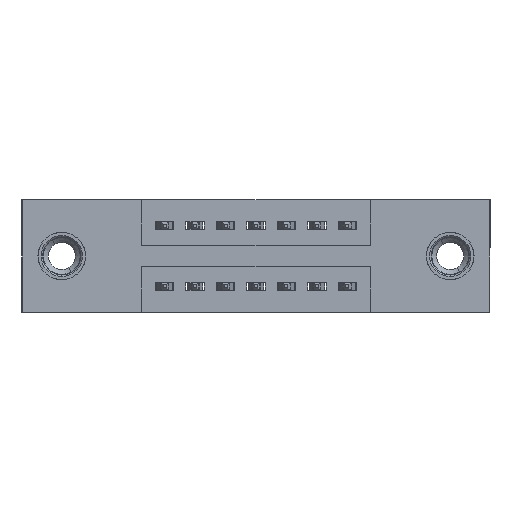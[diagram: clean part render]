
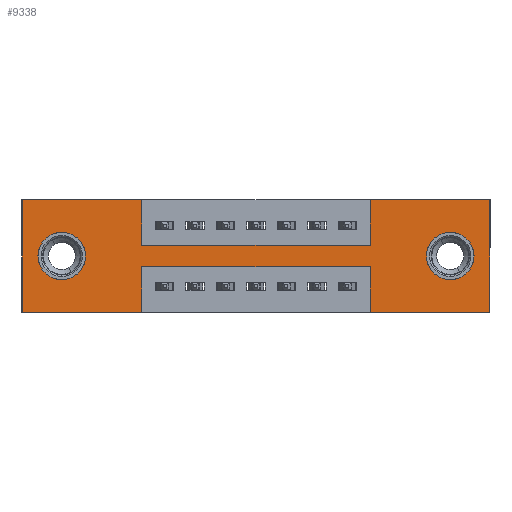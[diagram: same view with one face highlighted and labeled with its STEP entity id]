
A CAD part, front view. The second image highlights one B-rep face of the part: STEP entity #9338.
In plain terms, the highlighted planar face has unit normal (0, -1, 0).
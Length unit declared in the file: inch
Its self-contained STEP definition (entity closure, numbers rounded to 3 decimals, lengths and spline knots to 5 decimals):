
#310 = DIRECTION ( 'NONE',  ( 0., 1., 0. ) ) ;
#354 = LINE ( 'NONE', #8380, #3101 ) ;
#454 = CARTESIAN_POINT ( 'NONE',  ( 0.3925, 0., 0. ) ) ;
#519 = FACE_BOUND ( 'NONE', #1555, .T. ) ;
#572 = ORIENTED_EDGE ( 'NONE', *, *, #2110, .T. ) ;
#616 = CARTESIAN_POINT ( 'NONE',  ( 1.535, 0., -0.37 ) ) ;
#624 = LINE ( 'NONE', #11600, #9513 ) ;
#793 = VERTEX_POINT ( 'NONE', #9125 ) ;
#944 = ORIENTED_EDGE ( 'NONE', *, *, #11783, .F. ) ;
#978 = DIRECTION ( 'NONE',  ( 0., 1., 0. ) ) ;
#1040 = VERTEX_POINT ( 'NONE', #5684 ) ;
#1214 = DIRECTION ( 'NONE',  ( 0., 0., -1. ) ) ;
#1364 = AXIS2_PLACEMENT_3D ( 'NONE', #6795, #3445, #2253 ) ;
#1555 = EDGE_LOOP ( 'NONE', ( #9147, #572 ) ) ;
#1647 = VECTOR ( 'NONE', #11703, 39.37008 ) ;
#1664 = VECTOR ( 'NONE', #3648, 39.37008 ) ;
#1700 = CIRCLE ( 'NONE', #11660, 0.078 ) ;
#1796 = VERTEX_POINT ( 'NONE', #5261 ) ;
#1831 = CIRCLE ( 'NONE', #1364, 0.078 ) ;
#1840 = EDGE_CURVE ( 'NONE', #13525, #9590, #12715, .T. ) ;
#2037 = EDGE_CURVE ( 'NONE', #6480, #1040, #12182, .T. ) ;
#2058 = CARTESIAN_POINT ( 'NONE',  ( 0.13, 0., -0.185 ) ) ;
#2110 = EDGE_CURVE ( 'NONE', #3504, #793, #1831, .T. ) ;
#2253 = DIRECTION ( 'NONE',  ( 0., 0., -1. ) ) ;
#2272 = ORIENTED_EDGE ( 'NONE', *, *, #5285, .F. ) ;
#2352 = VECTOR ( 'NONE', #1214, 39.37008 ) ;
#2483 = ORIENTED_EDGE ( 'NONE', *, *, #1840, .F. ) ;
#2547 = ORIENTED_EDGE ( 'NONE', *, *, #14667, .F. ) ;
#2696 = VERTEX_POINT ( 'NONE', #13065 ) ;
#2777 = CARTESIAN_POINT ( 'NONE',  ( 0., 0., -0.37 ) ) ;
#3079 = DIRECTION ( 'NONE',  ( 0., 1., 0. ) ) ;
#3101 = VECTOR ( 'NONE', #11606, 39.37008 ) ;
#3163 = CARTESIAN_POINT ( 'NONE',  ( 0.3925, 0., -0.22 ) ) ;
#3194 = DIRECTION ( 'NONE',  ( 0., 0., -1. ) ) ;
#3234 = DIRECTION ( 'NONE',  ( 0., 0., 1. ) ) ;
#3445 = DIRECTION ( 'NONE',  ( 0., 1., 0. ) ) ;
#3475 = VECTOR ( 'NONE', #5201, 39.37008 ) ;
#3504 = VERTEX_POINT ( 'NONE', #3774 ) ;
#3574 = CARTESIAN_POINT ( 'NONE',  ( 1.1425, 0., 0. ) ) ;
#3644 = DIRECTION ( 'NONE',  ( -1., 0., 0. ) ) ;
#3648 = DIRECTION ( 'NONE',  ( 1., 0., 0. ) ) ;
#3651 = CARTESIAN_POINT ( 'NONE',  ( 1.535, 0., 0. ) ) ;
#3675 = VECTOR ( 'NONE', #5371, 39.37008 ) ;
#3748 = VERTEX_POINT ( 'NONE', #454 ) ;
#3774 = CARTESIAN_POINT ( 'NONE',  ( 1.405, 0., -0.263 ) ) ;
#3895 = CARTESIAN_POINT ( 'NONE',  ( 0.13, 0., -0.185 ) ) ;
#4017 = VECTOR ( 'NONE', #12720, 39.37008 ) ;
#4092 = VECTOR ( 'NONE', #9627, 39.37008 ) ;
#4129 = ORIENTED_EDGE ( 'NONE', *, *, #4266, .F. ) ;
#4266 = EDGE_CURVE ( 'NONE', #1796, #6480, #4285, .T. ) ;
#4283 = VECTOR ( 'NONE', #3194, 39.37008 ) ;
#4285 = LINE ( 'NONE', #3574, #9907 ) ;
#4526 = ORIENTED_EDGE ( 'NONE', *, *, #2037, .F. ) ;
#4536 = ORIENTED_EDGE ( 'NONE', *, *, #6891, .F. ) ;
#4721 = LINE ( 'NONE', #9426, #1647 ) ;
#4742 = DIRECTION ( 'NONE',  ( 0., 0., 1. ) ) ;
#4751 = CARTESIAN_POINT ( 'NONE',  ( 0.3925, 0., -0.15 ) ) ;
#4876 = ORIENTED_EDGE ( 'NONE', *, *, #11147, .F. ) ;
#4954 = CARTESIAN_POINT ( 'NONE',  ( 0.3925, 0., 0. ) ) ;
#5201 = DIRECTION ( 'NONE',  ( -1., 0., 0. ) ) ;
#5261 = CARTESIAN_POINT ( 'NONE',  ( 1.1425, 0., -0.15 ) ) ;
#5285 = EDGE_CURVE ( 'NONE', #11711, #9975, #624, .T. ) ;
#5316 = CARTESIAN_POINT ( 'NONE',  ( 0., 0., -0.37 ) ) ;
#5371 = DIRECTION ( 'NONE',  ( -1., 0., 0. ) ) ;
#5490 = LINE ( 'NONE', #9422, #1664 ) ;
#5585 = CARTESIAN_POINT ( 'NONE',  ( 0.3925, 0., -0.37 ) ) ;
#5684 = CARTESIAN_POINT ( 'NONE',  ( 1.535, 0., 0. ) ) ;
#5934 = LINE ( 'NONE', #4954, #4092 ) ;
#6211 = VERTEX_POINT ( 'NONE', #4751 ) ;
#6480 = VERTEX_POINT ( 'NONE', #14315 ) ;
#6487 = CARTESIAN_POINT ( 'NONE',  ( 0.3925, 0., -0.22 ) ) ;
#6502 = ORIENTED_EDGE ( 'NONE', *, *, #14547, .F. ) ;
#6778 = LINE ( 'NONE', #6487, #3675 ) ;
#6795 = CARTESIAN_POINT ( 'NONE',  ( 1.405, 0., -0.185 ) ) ;
#6891 = EDGE_CURVE ( 'NONE', #2696, #3748, #5490, .T. ) ;
#7025 = EDGE_LOOP ( 'NONE', ( #11475, #11392 ) ) ;
#7071 = FACE_OUTER_BOUND ( 'NONE', #9387, .T. ) ;
#7572 = DIRECTION ( 'NONE',  ( 0., 0., -1. ) ) ;
#7664 = VECTOR ( 'NONE', #14555, 39.37008 ) ;
#7741 = LINE ( 'NONE', #5585, #4283 ) ;
#7746 = CARTESIAN_POINT ( 'NONE',  ( 0., 0., -0.37 ) ) ;
#8075 = CARTESIAN_POINT ( 'NONE',  ( 0., 0., 0. ) ) ;
#8107 = ORIENTED_EDGE ( 'NONE', *, *, #14725, .F. ) ;
#8380 = CARTESIAN_POINT ( 'NONE',  ( 1.1425, 0., -0.37 ) ) ;
#8453 = PLANE ( 'NONE',  #10273 ) ;
#9057 = EDGE_CURVE ( 'NONE', #793, #3504, #14098, .T. ) ;
#9125 = CARTESIAN_POINT ( 'NONE',  ( 1.405, 0., -0.107 ) ) ;
#9147 = ORIENTED_EDGE ( 'NONE', *, *, #9057, .T. ) ;
#9164 = VERTEX_POINT ( 'NONE', #10458 ) ;
#9198 = AXIS2_PLACEMENT_3D ( 'NONE', #9988, #3079, #7572 ) ;
#9338 = ADVANCED_FACE ( 'NONE', ( #519, #12498, #7071 ), #8453, .T. ) ;
#9387 = EDGE_LOOP ( 'NONE', ( #944, #10819, #8107, #2483, #13957, #4526, #4129, #2547, #4876, #4536, #6502, #2272 ) ) ;
#9422 = CARTESIAN_POINT ( 'NONE',  ( 0., 0., 0. ) ) ;
#9426 = CARTESIAN_POINT ( 'NONE',  ( 0.3925, 0., -0.15 ) ) ;
#9513 = VECTOR ( 'NONE', #3644, 39.37008 ) ;
#9590 = VERTEX_POINT ( 'NONE', #11728 ) ;
#9627 = DIRECTION ( 'NONE',  ( 0., 0., -1. ) ) ;
#9780 = CARTESIAN_POINT ( 'NONE',  ( 0.13, 0., -0.107 ) ) ;
#9907 = VECTOR ( 'NONE', #4742, 39.37008 ) ;
#9947 = CARTESIAN_POINT ( 'NONE',  ( 0.3925, 0., -0.37 ) ) ;
#9975 = VERTEX_POINT ( 'NONE', #2777 ) ;
#9988 = CARTESIAN_POINT ( 'NONE',  ( 1.405, 0., -0.185 ) ) ;
#9998 = CARTESIAN_POINT ( 'NONE',  ( 0., 0., 0. ) ) ;
#10165 = LINE ( 'NONE', #8075, #4017 ) ;
#10273 = AXIS2_PLACEMENT_3D ( 'NONE', #7746, #11111, #11895 ) ;
#10458 = CARTESIAN_POINT ( 'NONE',  ( 1.1425, 0., -0.22 ) ) ;
#10794 = CARTESIAN_POINT ( 'NONE',  ( 0.13, 0., -0.263 ) ) ;
#10819 = ORIENTED_EDGE ( 'NONE', *, *, #13719, .F. ) ;
#11111 = DIRECTION ( 'NONE',  ( 0., -1., 0. ) ) ;
#11147 = EDGE_CURVE ( 'NONE', #3748, #6211, #5934, .T. ) ;
#11150 = CIRCLE ( 'NONE', #13580, 0.078 ) ;
#11392 = ORIENTED_EDGE ( 'NONE', *, *, #12456, .T. ) ;
#11438 = VERTEX_POINT ( 'NONE', #10794 ) ;
#11475 = ORIENTED_EDGE ( 'NONE', *, *, #12775, .T. ) ;
#11600 = CARTESIAN_POINT ( 'NONE',  ( 0., 0., -0.37 ) ) ;
#11606 = DIRECTION ( 'NONE',  ( 0., 0., 1. ) ) ;
#11660 = AXIS2_PLACEMENT_3D ( 'NONE', #3895, #310, #13146 ) ;
#11703 = DIRECTION ( 'NONE',  ( 1., 0., 0. ) ) ;
#11711 = VERTEX_POINT ( 'NONE', #9947 ) ;
#11728 = CARTESIAN_POINT ( 'NONE',  ( 1.1425, 0., -0.37 ) ) ;
#11783 = EDGE_CURVE ( 'NONE', #12340, #11711, #7741, .T. ) ;
#11895 = DIRECTION ( 'NONE',  ( 0., 0., -1. ) ) ;
#12067 = VERTEX_POINT ( 'NONE', #9780 ) ;
#12182 = LINE ( 'NONE', #9998, #7664 ) ;
#12340 = VERTEX_POINT ( 'NONE', #3163 ) ;
#12456 = EDGE_CURVE ( 'NONE', #11438, #12067, #11150, .T. ) ;
#12498 = FACE_BOUND ( 'NONE', #7025, .T. ) ;
#12715 = LINE ( 'NONE', #5316, #3475 ) ;
#12720 = DIRECTION ( 'NONE',  ( 0., 0., 1. ) ) ;
#12775 = EDGE_CURVE ( 'NONE', #12067, #11438, #1700, .T. ) ;
#13065 = CARTESIAN_POINT ( 'NONE',  ( 0., 0., 0. ) ) ;
#13146 = DIRECTION ( 'NONE',  ( 0., 0., 1. ) ) ;
#13525 = VERTEX_POINT ( 'NONE', #616 ) ;
#13580 = AXIS2_PLACEMENT_3D ( 'NONE', #2058, #978, #3234 ) ;
#13719 = EDGE_CURVE ( 'NONE', #9164, #12340, #6778, .T. ) ;
#13945 = LINE ( 'NONE', #3651, #2352 ) ;
#13957 = ORIENTED_EDGE ( 'NONE', *, *, #14665, .F. ) ;
#14098 = CIRCLE ( 'NONE', #9198, 0.078 ) ;
#14315 = CARTESIAN_POINT ( 'NONE',  ( 1.1425, 0., 0. ) ) ;
#14547 = EDGE_CURVE ( 'NONE', #9975, #2696, #10165, .T. ) ;
#14555 = DIRECTION ( 'NONE',  ( 1., 0., 0. ) ) ;
#14665 = EDGE_CURVE ( 'NONE', #1040, #13525, #13945, .T. ) ;
#14667 = EDGE_CURVE ( 'NONE', #6211, #1796, #4721, .T. ) ;
#14725 = EDGE_CURVE ( 'NONE', #9590, #9164, #354, .T. ) ;
